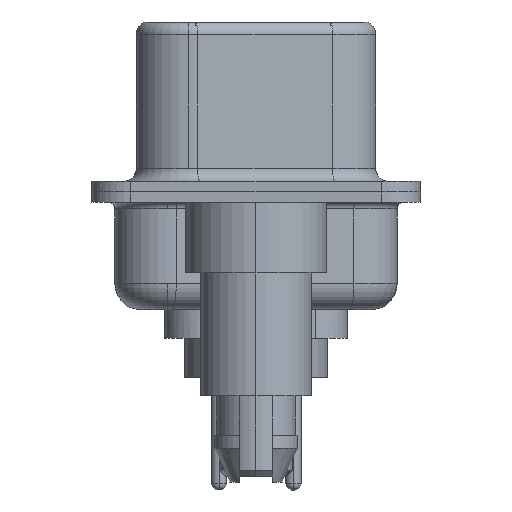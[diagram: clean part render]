
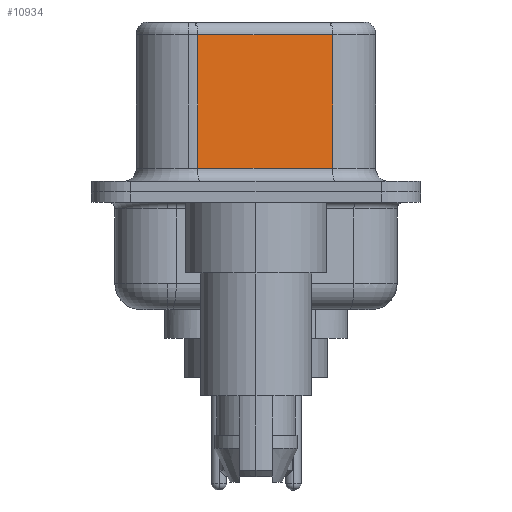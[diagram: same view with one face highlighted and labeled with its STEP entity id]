
A CAD part, left-side view. The second image highlights one B-rep face of the part: STEP entity #10934.
In plain terms, the highlighted planar face has unit normal (-0.985, -0.174, 0).
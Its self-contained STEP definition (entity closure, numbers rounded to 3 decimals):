
#1249 = LINE ( 'NONE', #3152, #20557 ) ;
#1444 = VECTOR ( 'NONE', #20645, 1000. ) ;
#1484 = CARTESIAN_POINT ( 'NONE',  ( 4.58, -2.927, 6.52 ) ) ;
#1526 = LINE ( 'NONE', #5223, #5964 ) ;
#3004 = AXIS2_PLACEMENT_3D ( 'NONE', #1484, #7179, #20217 ) ;
#3152 = CARTESIAN_POINT ( 'NONE',  ( 4.58, -2.927, 6.02 ) ) ;
#3732 = CARTESIAN_POINT ( 'NONE',  ( 4.58, -2.927, 0.9 ) ) ;
#4278 = EDGE_CURVE ( 'NONE', #20090, #13197, #1249, .T. ) ;
#5223 = CARTESIAN_POINT ( 'NONE',  ( 3.67, 2.233, 6.52 ) ) ;
#5430 = VERTEX_POINT ( 'NONE', #19115 ) ;
#5964 = VECTOR ( 'NONE', #10858, 1000. ) ;
#6294 = CARTESIAN_POINT ( 'NONE',  ( 4.58, -2.927, 6.02 ) ) ;
#6351 = ORIENTED_EDGE ( 'NONE', *, *, #12476, .F. ) ;
#6858 = ORIENTED_EDGE ( 'NONE', *, *, #4278, .T. ) ;
#6885 = ORIENTED_EDGE ( 'NONE', *, *, #10200, .T. ) ;
#7179 = DIRECTION ( 'NONE',  ( 0.985, 0.174, 0. ) ) ;
#7226 = ORIENTED_EDGE ( 'NONE', *, *, #21237, .T. ) ;
#7798 = CARTESIAN_POINT ( 'NONE',  ( 4.58, -2.927, 0.9 ) ) ;
#10200 = EDGE_CURVE ( 'NONE', #13197, #5430, #1526, .T. ) ;
#10858 = DIRECTION ( 'NONE',  ( 0., 0., -1. ) ) ;
#10934 = ADVANCED_FACE ( 'NONE', ( #18454 ), #18313, .F. ) ;
#12167 = EDGE_LOOP ( 'NONE', ( #6351, #6858, #6885, #7226 ) ) ;
#12476 = EDGE_CURVE ( 'NONE', #20090, #14868, #16404, .T. ) ;
#13197 = VERTEX_POINT ( 'NONE', #24133 ) ;
#14868 = VERTEX_POINT ( 'NONE', #3732 ) ;
#15317 = DIRECTION ( 'NONE',  ( 0.174, -0.985, 0. ) ) ;
#15977 = VECTOR ( 'NONE', #15317, 1000. ) ;
#16404 = LINE ( 'NONE', #18716, #1444 ) ;
#18313 = PLANE ( 'NONE',  #3004 ) ;
#18454 = FACE_OUTER_BOUND ( 'NONE', #12167, .T. ) ;
#18716 = CARTESIAN_POINT ( 'NONE',  ( 4.58, -2.927, 6.52 ) ) ;
#19115 = CARTESIAN_POINT ( 'NONE',  ( 3.67, 2.233, 0.9 ) ) ;
#20090 = VERTEX_POINT ( 'NONE', #6294 ) ;
#20217 = DIRECTION ( 'NONE',  ( -0.174, 0.985, 0. ) ) ;
#20557 = VECTOR ( 'NONE', #23186, 1000. ) ;
#20645 = DIRECTION ( 'NONE',  ( 0., 0., -1. ) ) ;
#20943 = LINE ( 'NONE', #7798, #15977 ) ;
#21237 = EDGE_CURVE ( 'NONE', #5430, #14868, #20943, .T. ) ;
#23186 = DIRECTION ( 'NONE',  ( -0.174, 0.985, 0. ) ) ;
#24133 = CARTESIAN_POINT ( 'NONE',  ( 3.67, 2.233, 6.02 ) ) ;
